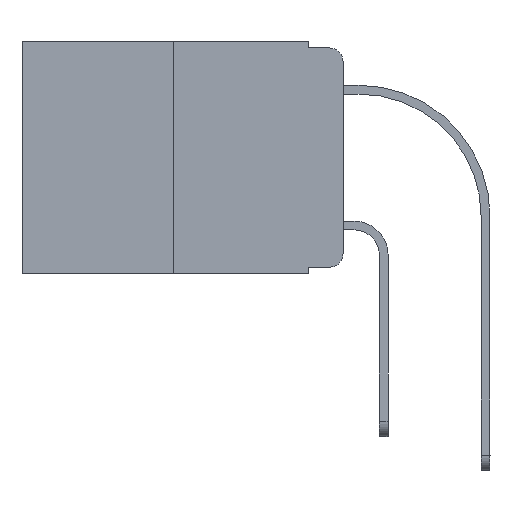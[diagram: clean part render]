
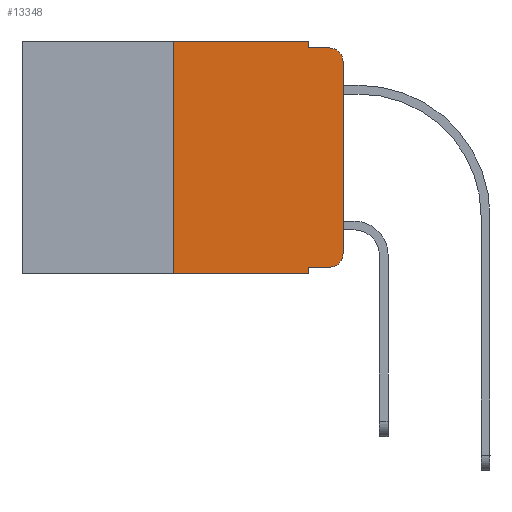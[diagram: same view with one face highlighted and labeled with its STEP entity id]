
A CAD part, left-side view. The second image highlights one B-rep face of the part: STEP entity #13348.
In plain terms, the highlighted planar face has unit normal (-1, 0, 0).
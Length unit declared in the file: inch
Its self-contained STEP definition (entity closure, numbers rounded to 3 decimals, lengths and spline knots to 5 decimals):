
#5 = EDGE_CURVE ( 'NONE', #13998, #4227, #5480, .T. ) ;
#302 = DIRECTION ( 'NONE',  ( 0., -1., 0. ) ) ;
#306 = CIRCLE ( 'NONE', #13430, 0.02 ) ;
#331 = DIRECTION ( 'NONE',  ( 0., 0., -1. ) ) ;
#573 = DIRECTION ( 'NONE',  ( 0., 0., -1. ) ) ;
#704 = VERTEX_POINT ( 'NONE', #11952 ) ;
#980 = VECTOR ( 'NONE', #10831, 39.37008 ) ;
#1308 = LINE ( 'NONE', #19032, #18576 ) ;
#1770 = VERTEX_POINT ( 'NONE', #14645 ) ;
#2118 = DIRECTION ( 'NONE',  ( 0., -1., 0. ) ) ;
#2196 = EDGE_CURVE ( 'NONE', #4227, #704, #13985, .T. ) ;
#2205 = ORIENTED_EDGE ( 'NONE', *, *, #4755, .T. ) ;
#2250 = CARTESIAN_POINT ( 'NONE',  ( 0., 0.051, -0.343 ) ) ;
#2354 = ORIENTED_EDGE ( 'NONE', *, *, #6817, .F. ) ;
#2498 = CARTESIAN_POINT ( 'NONE',  ( 0., 0.051, -0.01 ) ) ;
#2529 = VECTOR ( 'NONE', #302, 39.37008 ) ;
#3343 = ORIENTED_EDGE ( 'NONE', *, *, #8930, .F. ) ;
#3367 = EDGE_CURVE ( 'NONE', #12639, #13998, #306, .T. ) ;
#3461 = VERTEX_POINT ( 'NONE', #4979 ) ;
#3698 = VERTEX_POINT ( 'NONE', #17408 ) ;
#3703 = CARTESIAN_POINT ( 'NONE',  ( 0., 0.02, -0.313 ) ) ;
#3746 = EDGE_CURVE ( 'NONE', #3698, #12639, #11250, .T. ) ;
#3849 = CARTESIAN_POINT ( 'NONE',  ( 0., 0.473, 0. ) ) ;
#4227 = VERTEX_POINT ( 'NONE', #13259 ) ;
#4461 = LINE ( 'NONE', #13862, #11663 ) ;
#4755 = EDGE_CURVE ( 'NONE', #1770, #13821, #14488, .T. ) ;
#4979 = CARTESIAN_POINT ( 'NONE',  ( 0., 0.051, -0.01 ) ) ;
#5252 = CARTESIAN_POINT ( 'NONE',  ( 0., 0.25, 0. ) ) ;
#5480 = LINE ( 'NONE', #8426, #7970 ) ;
#5828 = EDGE_CURVE ( 'NONE', #1770, #10148, #13139, .T. ) ;
#6515 = LINE ( 'NONE', #9782, #2529 ) ;
#6817 = EDGE_CURVE ( 'NONE', #3461, #704, #9777, .T. ) ;
#6993 = EDGE_LOOP ( 'NONE', ( #10504, #15121, #2354, #3343, #14818, #18176, #2205, #9448, #17744, #16136 ) ) ;
#7734 = DIRECTION ( 'NONE',  ( 0., 0., -1. ) ) ;
#7970 = VECTOR ( 'NONE', #13483, 39.37008 ) ;
#8426 = CARTESIAN_POINT ( 'NONE',  ( 0., 0., 0. ) ) ;
#8549 = DIRECTION ( 'NONE',  ( -1., 0., 0. ) ) ;
#8744 = VERTEX_POINT ( 'NONE', #11206 ) ;
#8930 = EDGE_CURVE ( 'NONE', #8744, #3461, #4461, .T. ) ;
#9141 = DIRECTION ( 'NONE',  ( 0., -1., 0. ) ) ;
#9215 = AXIS2_PLACEMENT_3D ( 'NONE', #3849, #20312, #19997 ) ;
#9448 = ORIENTED_EDGE ( 'NONE', *, *, #16370, .F. ) ;
#9678 = VECTOR ( 'NONE', #2118, 39.37008 ) ;
#9753 = DIRECTION ( 'NONE',  ( 0., 0., 1. ) ) ;
#9777 = LINE ( 'NONE', #2498, #19965 ) ;
#9782 = CARTESIAN_POINT ( 'NONE',  ( 0., 0.473, 0. ) ) ;
#10062 = CARTESIAN_POINT ( 'NONE',  ( 0., 0.02, -0.03 ) ) ;
#10148 = VERTEX_POINT ( 'NONE', #5252 ) ;
#10504 = ORIENTED_EDGE ( 'NONE', *, *, #5, .T. ) ;
#10831 = DIRECTION ( 'NONE',  ( 0., -1., 0. ) ) ;
#11206 = CARTESIAN_POINT ( 'NONE',  ( 0., 0.051, 0. ) ) ;
#11250 = LINE ( 'NONE', #14323, #980 ) ;
#11315 = EDGE_CURVE ( 'NONE', #10148, #8744, #6515, .T. ) ;
#11663 = VECTOR ( 'NONE', #20515, 39.37008 ) ;
#11947 = PLANE ( 'NONE',  #9215 ) ;
#11952 = CARTESIAN_POINT ( 'NONE',  ( 0., 0.02, -0.01 ) ) ;
#12639 = VERTEX_POINT ( 'NONE', #17705 ) ;
#13139 = LINE ( 'NONE', #14918, #17894 ) ;
#13259 = CARTESIAN_POINT ( 'NONE',  ( 0., 0., -0.03 ) ) ;
#13348 = ADVANCED_FACE ( 'NONE', ( #13460 ), #11947, .F. ) ;
#13430 = AXIS2_PLACEMENT_3D ( 'NONE', #3703, #8549, #331 ) ;
#13460 = FACE_OUTER_BOUND ( 'NONE', #6993, .T. ) ;
#13483 = DIRECTION ( 'NONE',  ( 0., 0., 1. ) ) ;
#13821 = VERTEX_POINT ( 'NONE', #2250 ) ;
#13862 = CARTESIAN_POINT ( 'NONE',  ( 0., 0.051, 0. ) ) ;
#13985 = CIRCLE ( 'NONE', #16349, 0.02 ) ;
#13998 = VERTEX_POINT ( 'NONE', #17133 ) ;
#14323 = CARTESIAN_POINT ( 'NONE',  ( 0., 0.051, -0.333 ) ) ;
#14488 = LINE ( 'NONE', #16578, #9678 ) ;
#14645 = CARTESIAN_POINT ( 'NONE',  ( 0., 0.25, -0.343 ) ) ;
#14818 = ORIENTED_EDGE ( 'NONE', *, *, #11315, .F. ) ;
#14918 = CARTESIAN_POINT ( 'NONE',  ( 0., 0.25, 0. ) ) ;
#15024 = DIRECTION ( 'NONE',  ( -1., 0., 0. ) ) ;
#15121 = ORIENTED_EDGE ( 'NONE', *, *, #2196, .T. ) ;
#16136 = ORIENTED_EDGE ( 'NONE', *, *, #3367, .T. ) ;
#16349 = AXIS2_PLACEMENT_3D ( 'NONE', #10062, #15024, #573 ) ;
#16370 = EDGE_CURVE ( 'NONE', #3698, #13821, #1308, .T. ) ;
#16578 = CARTESIAN_POINT ( 'NONE',  ( 0., 0.473, -0.343 ) ) ;
#17133 = CARTESIAN_POINT ( 'NONE',  ( 0., 0., -0.313 ) ) ;
#17408 = CARTESIAN_POINT ( 'NONE',  ( 0., 0.051, -0.333 ) ) ;
#17705 = CARTESIAN_POINT ( 'NONE',  ( 0., 0.02, -0.333 ) ) ;
#17744 = ORIENTED_EDGE ( 'NONE', *, *, #3746, .T. ) ;
#17894 = VECTOR ( 'NONE', #9753, 39.37008 ) ;
#18176 = ORIENTED_EDGE ( 'NONE', *, *, #5828, .F. ) ;
#18576 = VECTOR ( 'NONE', #7734, 39.37008 ) ;
#19032 = CARTESIAN_POINT ( 'NONE',  ( 0., 0.051, 0. ) ) ;
#19965 = VECTOR ( 'NONE', #9141, 39.37008 ) ;
#19997 = DIRECTION ( 'NONE',  ( 0., 0., -1. ) ) ;
#20312 = DIRECTION ( 'NONE',  ( 1., 0., 0. ) ) ;
#20515 = DIRECTION ( 'NONE',  ( 0., 0., -1. ) ) ;
